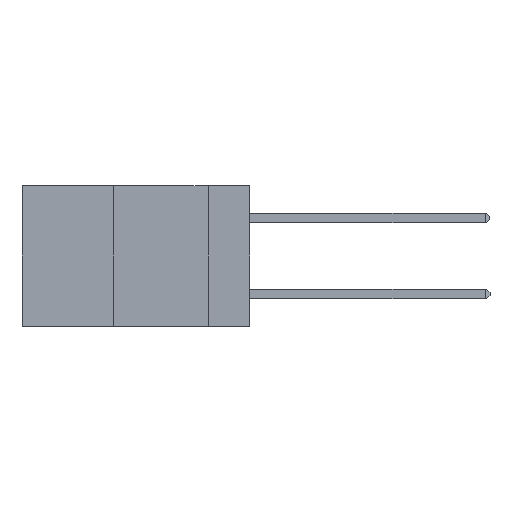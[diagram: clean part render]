
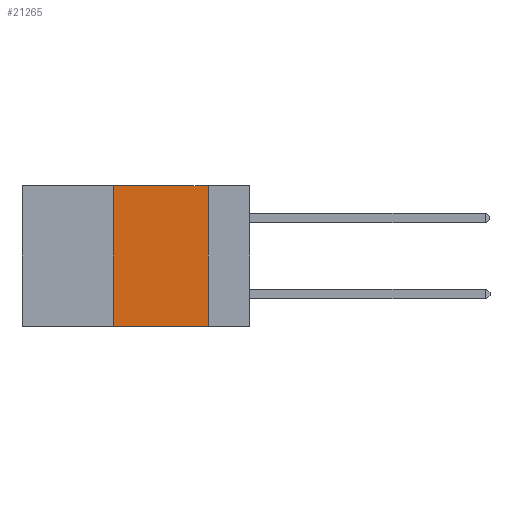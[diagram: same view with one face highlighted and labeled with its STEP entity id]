
A CAD part, left-side view. The second image highlights one B-rep face of the part: STEP entity #21265.
In plain terms, the highlighted planar face has unit normal (-1, 0, 0).
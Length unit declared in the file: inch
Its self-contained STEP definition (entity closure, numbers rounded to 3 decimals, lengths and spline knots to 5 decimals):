
#87 = ORIENTED_EDGE ( 'NONE', *, *, #8526, .F. ) ;
#178 = EDGE_CURVE ( 'NONE', #16048, #5520, #5963, .T. ) ;
#493 = VERTEX_POINT ( 'NONE', #14710 ) ;
#524 = EDGE_CURVE ( 'NONE', #5520, #20391, #14121, .T. ) ;
#866 = ORIENTED_EDGE ( 'NONE', *, *, #5613, .T. ) ;
#1019 = VECTOR ( 'NONE', #5595, 39.37008 ) ;
#1230 = CARTESIAN_POINT ( 'NONE',  ( 0., 0.36, 0. ) ) ;
#1422 = DIRECTION ( 'NONE',  ( 0., 0., -1. ) ) ;
#2613 = VECTOR ( 'NONE', #18253, 39.37008 ) ;
#2708 = EDGE_LOOP ( 'NONE', ( #5714, #6166, #87, #866 ) ) ;
#4299 = FACE_OUTER_BOUND ( 'NONE', #2708, .T. ) ;
#4959 = CARTESIAN_POINT ( 'NONE',  ( 0., 0.11, -0.37 ) ) ;
#5219 = CARTESIAN_POINT ( 'NONE',  ( 0., 0.6, -0.37 ) ) ;
#5520 = VERTEX_POINT ( 'NONE', #13145 ) ;
#5595 = DIRECTION ( 'NONE',  ( 0., -1., 0. ) ) ;
#5613 = EDGE_CURVE ( 'NONE', #493, #20391, #14796, .T. ) ;
#5714 = ORIENTED_EDGE ( 'NONE', *, *, #524, .F. ) ;
#5846 = PLANE ( 'NONE',  #12371 ) ;
#5963 = LINE ( 'NONE', #16620, #1019 ) ;
#6082 = VECTOR ( 'NONE', #18350, 39.37008 ) ;
#6166 = ORIENTED_EDGE ( 'NONE', *, *, #178, .F. ) ;
#6840 = CARTESIAN_POINT ( 'NONE',  ( 0., 0.36, 0. ) ) ;
#7508 = CARTESIAN_POINT ( 'NONE',  ( 0., 0.6, 0. ) ) ;
#8526 = EDGE_CURVE ( 'NONE', #493, #16048, #15498, .T. ) ;
#9142 = DIRECTION ( 'NONE',  ( 0., 0., -1. ) ) ;
#12371 = AXIS2_PLACEMENT_3D ( 'NONE', #7508, #18958, #9142 ) ;
#13145 = CARTESIAN_POINT ( 'NONE',  ( 0., 0.11, 0. ) ) ;
#13623 = VECTOR ( 'NONE', #1422, 39.37008 ) ;
#14121 = LINE ( 'NONE', #20661, #13623 ) ;
#14710 = CARTESIAN_POINT ( 'NONE',  ( 0., 0.36, -0.37 ) ) ;
#14796 = LINE ( 'NONE', #5219, #6082 ) ;
#15498 = LINE ( 'NONE', #6840, #2613 ) ;
#16048 = VERTEX_POINT ( 'NONE', #1230 ) ;
#16620 = CARTESIAN_POINT ( 'NONE',  ( 0., 0.6, 0. ) ) ;
#18253 = DIRECTION ( 'NONE',  ( 0., 0., 1. ) ) ;
#18350 = DIRECTION ( 'NONE',  ( 0., -1., 0. ) ) ;
#18958 = DIRECTION ( 'NONE',  ( 1., 0., 0. ) ) ;
#20391 = VERTEX_POINT ( 'NONE', #4959 ) ;
#20661 = CARTESIAN_POINT ( 'NONE',  ( 0., 0.11, 0. ) ) ;
#21265 = ADVANCED_FACE ( 'NONE', ( #4299 ), #5846, .F. ) ;
